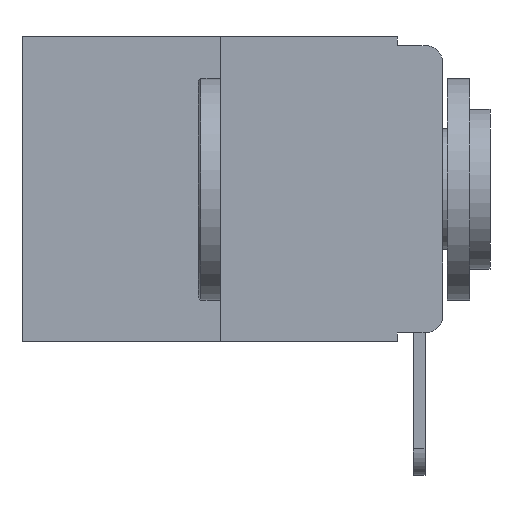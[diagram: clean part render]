
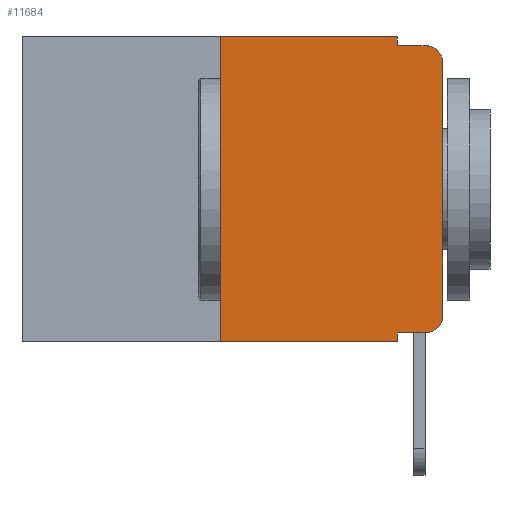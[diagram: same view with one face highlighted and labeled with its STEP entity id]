
A CAD part, left-side view. The second image highlights one B-rep face of the part: STEP entity #11684.
In plain terms, the highlighted planar face has unit normal (-1, 0, 0).
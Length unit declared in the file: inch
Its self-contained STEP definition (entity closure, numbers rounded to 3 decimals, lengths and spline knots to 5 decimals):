
#305 = VECTOR ( 'NONE', #3589, 39.37008 ) ;
#657 = VECTOR ( 'NONE', #6342, 39.37008 ) ;
#1008 = ORIENTED_EDGE ( 'NONE', *, *, #9051, .T. ) ;
#1134 = DIRECTION ( 'NONE',  ( 0., 0., -1. ) ) ;
#1397 = CARTESIAN_POINT ( 'NONE',  ( 0., 0.473, 0. ) ) ;
#1480 = ORIENTED_EDGE ( 'NONE', *, *, #5508, .F. ) ;
#1758 = DIRECTION ( 'NONE',  ( -1., 0., 0. ) ) ;
#1807 = CARTESIAN_POINT ( 'NONE',  ( 0., 0., -0.313 ) ) ;
#2033 = AXIS2_PLACEMENT_3D ( 'NONE', #8432, #1758, #9427 ) ;
#2392 = VERTEX_POINT ( 'NONE', #9464 ) ;
#2433 = DIRECTION ( 'NONE',  ( 0., -1., 0. ) ) ;
#2499 = DIRECTION ( 'NONE',  ( -1., 0., 0. ) ) ;
#2819 = AXIS2_PLACEMENT_3D ( 'NONE', #13495, #7961, #1134 ) ;
#2861 = CARTESIAN_POINT ( 'NONE',  ( 0., 0.051, -0.01 ) ) ;
#2900 = FACE_OUTER_BOUND ( 'NONE', #11465, .T. ) ;
#2957 = CARTESIAN_POINT ( 'NONE',  ( 0., 0.051, 0. ) ) ;
#2978 = ORIENTED_EDGE ( 'NONE', *, *, #13184, .T. ) ;
#3021 = VECTOR ( 'NONE', #13147, 39.37008 ) ;
#3233 = VERTEX_POINT ( 'NONE', #1807 ) ;
#3260 = ORIENTED_EDGE ( 'NONE', *, *, #13301, .F. ) ;
#3428 = CARTESIAN_POINT ( 'NONE',  ( 0., 0.473, -0.343 ) ) ;
#3514 = AXIS2_PLACEMENT_3D ( 'NONE', #9039, #2499, #10013 ) ;
#3588 = EDGE_CURVE ( 'NONE', #9747, #8776, #5983, .T. ) ;
#3589 = DIRECTION ( 'NONE',  ( 0., 0., 1. ) ) ;
#4084 = CARTESIAN_POINT ( 'NONE',  ( 0., 0.051, 0. ) ) ;
#4129 = VERTEX_POINT ( 'NONE', #8941 ) ;
#4367 = LINE ( 'NONE', #2861, #657 ) ;
#4607 = CARTESIAN_POINT ( 'NONE',  ( 0., 0.051, -0.343 ) ) ;
#5146 = VERTEX_POINT ( 'NONE', #5895 ) ;
#5363 = CARTESIAN_POINT ( 'NONE',  ( 0., 0., 0. ) ) ;
#5429 = ORIENTED_EDGE ( 'NONE', *, *, #10776, .T. ) ;
#5508 = EDGE_CURVE ( 'NONE', #5146, #6765, #7584, .T. ) ;
#5587 = VECTOR ( 'NONE', #9454, 39.37008 ) ;
#5747 = CARTESIAN_POINT ( 'NONE',  ( 0., 0.25, -0.343 ) ) ;
#5895 = CARTESIAN_POINT ( 'NONE',  ( 0., 0.25, 0. ) ) ;
#5983 = LINE ( 'NONE', #13262, #12977 ) ;
#6342 = DIRECTION ( 'NONE',  ( 0., -1., 0. ) ) ;
#6668 = CARTESIAN_POINT ( 'NONE',  ( 0., 0.051, -0.333 ) ) ;
#6765 = VERTEX_POINT ( 'NONE', #2957 ) ;
#6800 = LINE ( 'NONE', #12280, #3021 ) ;
#7413 = EDGE_CURVE ( 'NONE', #2392, #10302, #4367, .T. ) ;
#7584 = LINE ( 'NONE', #1397, #7911 ) ;
#7792 = VERTEX_POINT ( 'NONE', #4607 ) ;
#7911 = VECTOR ( 'NONE', #8878, 39.37008 ) ;
#7961 = DIRECTION ( 'NONE',  ( 1., 0., 0. ) ) ;
#8294 = LINE ( 'NONE', #5363, #5587 ) ;
#8432 = CARTESIAN_POINT ( 'NONE',  ( 0., 0.02, -0.313 ) ) ;
#8569 = CIRCLE ( 'NONE', #3514, 0.02 ) ;
#8676 = CARTESIAN_POINT ( 'NONE',  ( 0., 0.02, -0.01 ) ) ;
#8776 = VERTEX_POINT ( 'NONE', #9266 ) ;
#8878 = DIRECTION ( 'NONE',  ( 0., -1., 0. ) ) ;
#8941 = CARTESIAN_POINT ( 'NONE',  ( 0., 0., -0.03 ) ) ;
#8959 = ORIENTED_EDGE ( 'NONE', *, *, #9458, .F. ) ;
#9039 = CARTESIAN_POINT ( 'NONE',  ( 0., 0.02, -0.03 ) ) ;
#9051 = EDGE_CURVE ( 'NONE', #3233, #4129, #8294, .T. ) ;
#9266 = CARTESIAN_POINT ( 'NONE',  ( 0., 0.02, -0.333 ) ) ;
#9365 = LINE ( 'NONE', #9915, #305 ) ;
#9373 = LINE ( 'NONE', #4084, #13594 ) ;
#9427 = DIRECTION ( 'NONE',  ( 0., 0., -1. ) ) ;
#9454 = DIRECTION ( 'NONE',  ( 0., 0., 1. ) ) ;
#9458 = EDGE_CURVE ( 'NONE', #6765, #2392, #9373, .T. ) ;
#9464 = CARTESIAN_POINT ( 'NONE',  ( 0., 0.051, -0.01 ) ) ;
#9477 = ORIENTED_EDGE ( 'NONE', *, *, #3588, .T. ) ;
#9733 = ORIENTED_EDGE ( 'NONE', *, *, #9873, .T. ) ;
#9747 = VERTEX_POINT ( 'NONE', #6668 ) ;
#9873 = EDGE_CURVE ( 'NONE', #12614, #7792, #12645, .T. ) ;
#9915 = CARTESIAN_POINT ( 'NONE',  ( 0., 0.25, 0. ) ) ;
#9999 = EDGE_CURVE ( 'NONE', #12614, #5146, #9365, .T. ) ;
#10013 = DIRECTION ( 'NONE',  ( 0., 0., -1. ) ) ;
#10240 = DIRECTION ( 'NONE',  ( 0., 0., -1. ) ) ;
#10247 = VECTOR ( 'NONE', #11673, 39.37008 ) ;
#10302 = VERTEX_POINT ( 'NONE', #8676 ) ;
#10331 = CIRCLE ( 'NONE', #2033, 0.02 ) ;
#10776 = EDGE_CURVE ( 'NONE', #4129, #10302, #8569, .T. ) ;
#11465 = EDGE_LOOP ( 'NONE', ( #1008, #5429, #13618, #8959, #1480, #13385, #9733, #3260, #9477, #2978 ) ) ;
#11673 = DIRECTION ( 'NONE',  ( 0., -1., 0. ) ) ;
#11684 = ADVANCED_FACE ( 'NONE', ( #2900 ), #11787, .F. ) ;
#11787 = PLANE ( 'NONE',  #2819 ) ;
#12280 = CARTESIAN_POINT ( 'NONE',  ( 0., 0.051, 0. ) ) ;
#12614 = VERTEX_POINT ( 'NONE', #5747 ) ;
#12645 = LINE ( 'NONE', #3428, #10247 ) ;
#12977 = VECTOR ( 'NONE', #2433, 39.37008 ) ;
#13147 = DIRECTION ( 'NONE',  ( 0., 0., -1. ) ) ;
#13184 = EDGE_CURVE ( 'NONE', #8776, #3233, #10331, .T. ) ;
#13262 = CARTESIAN_POINT ( 'NONE',  ( 0., 0.051, -0.333 ) ) ;
#13301 = EDGE_CURVE ( 'NONE', #9747, #7792, #6800, .T. ) ;
#13385 = ORIENTED_EDGE ( 'NONE', *, *, #9999, .F. ) ;
#13495 = CARTESIAN_POINT ( 'NONE',  ( 0., 0.473, 0. ) ) ;
#13594 = VECTOR ( 'NONE', #10240, 39.37008 ) ;
#13618 = ORIENTED_EDGE ( 'NONE', *, *, #7413, .F. ) ;
